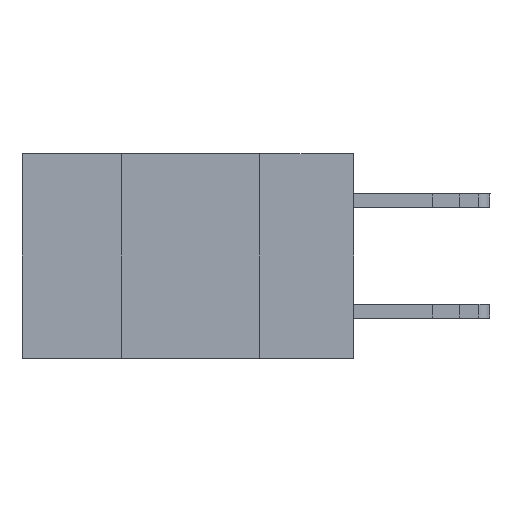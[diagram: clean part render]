
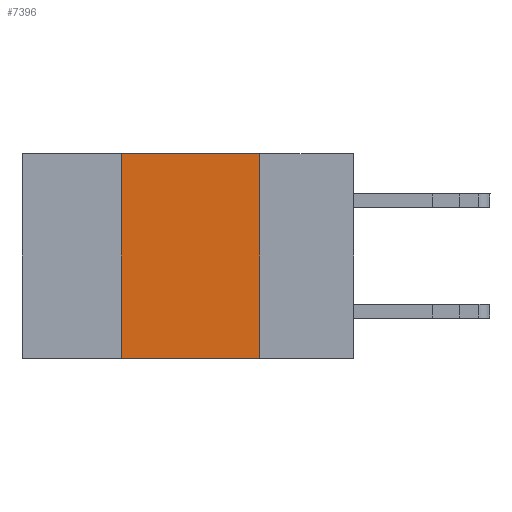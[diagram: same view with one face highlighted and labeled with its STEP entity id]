
A CAD part, left-side view. The second image highlights one B-rep face of the part: STEP entity #7396.
In plain terms, the highlighted planar face has unit normal (-1, 0, 0).
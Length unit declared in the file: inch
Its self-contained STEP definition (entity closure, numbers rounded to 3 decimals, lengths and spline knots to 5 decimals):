
#2838 = EDGE_CURVE ( 'NONE', #22701, #15177, #24760, .T. ) ;
#2873 = CARTESIAN_POINT ( 'NONE',  ( 0., 0.17, 0. ) ) ;
#3092 = LINE ( 'NONE', #24115, #7904 ) ;
#3538 = DIRECTION ( 'NONE',  ( 0., 0., 1. ) ) ;
#3614 = CARTESIAN_POINT ( 'NONE',  ( 0., 0.6, -0.37 ) ) ;
#3746 = CARTESIAN_POINT ( 'NONE',  ( 0., 0.17, 0. ) ) ;
#4698 = VECTOR ( 'NONE', #24705, 39.37008 ) ;
#5286 = CARTESIAN_POINT ( 'NONE',  ( 0., 0.6, 0. ) ) ;
#5539 = DIRECTION ( 'NONE',  ( 0., -1., 0. ) ) ;
#7081 = DIRECTION ( 'NONE',  ( 0., 0., -1. ) ) ;
#7396 = ADVANCED_FACE ( 'NONE', ( #19568 ), #18677, .F. ) ;
#7440 = EDGE_CURVE ( 'NONE', #23670, #15177, #10155, .T. ) ;
#7462 = VECTOR ( 'NONE', #14652, 39.37008 ) ;
#7904 = VECTOR ( 'NONE', #3538, 39.37008 ) ;
#7961 = AXIS2_PLACEMENT_3D ( 'NONE', #5286, #11310, #7081 ) ;
#8592 = ORIENTED_EDGE ( 'NONE', *, *, #2838, .F. ) ;
#9116 = ORIENTED_EDGE ( 'NONE', *, *, #9606, .F. ) ;
#9606 = EDGE_CURVE ( 'NONE', #23670, #10859, #3092, .T. ) ;
#10155 = LINE ( 'NONE', #3614, #18988 ) ;
#10859 = VERTEX_POINT ( 'NONE', #14629 ) ;
#11139 = CARTESIAN_POINT ( 'NONE',  ( 0., 0.6, 0. ) ) ;
#11310 = DIRECTION ( 'NONE',  ( 1., 0., 0. ) ) ;
#12037 = EDGE_LOOP ( 'NONE', ( #8592, #14494, #9116, #17142 ) ) ;
#12241 = CARTESIAN_POINT ( 'NONE',  ( 0., 0.17, -0.37 ) ) ;
#13661 = EDGE_CURVE ( 'NONE', #10859, #22701, #15040, .T. ) ;
#13859 = CARTESIAN_POINT ( 'NONE',  ( 0., 0.42, -0.37 ) ) ;
#14494 = ORIENTED_EDGE ( 'NONE', *, *, #13661, .F. ) ;
#14629 = CARTESIAN_POINT ( 'NONE',  ( 0., 0.42, 0. ) ) ;
#14652 = DIRECTION ( 'NONE',  ( 0., 0., -1. ) ) ;
#15040 = LINE ( 'NONE', #11139, #4698 ) ;
#15177 = VERTEX_POINT ( 'NONE', #12241 ) ;
#17142 = ORIENTED_EDGE ( 'NONE', *, *, #7440, .T. ) ;
#18677 = PLANE ( 'NONE',  #7961 ) ;
#18988 = VECTOR ( 'NONE', #5539, 39.37008 ) ;
#19568 = FACE_OUTER_BOUND ( 'NONE', #12037, .T. ) ;
#22701 = VERTEX_POINT ( 'NONE', #3746 ) ;
#23670 = VERTEX_POINT ( 'NONE', #13859 ) ;
#24115 = CARTESIAN_POINT ( 'NONE',  ( 0., 0.42, 0. ) ) ;
#24705 = DIRECTION ( 'NONE',  ( 0., -1., 0. ) ) ;
#24760 = LINE ( 'NONE', #2873, #7462 ) ;
